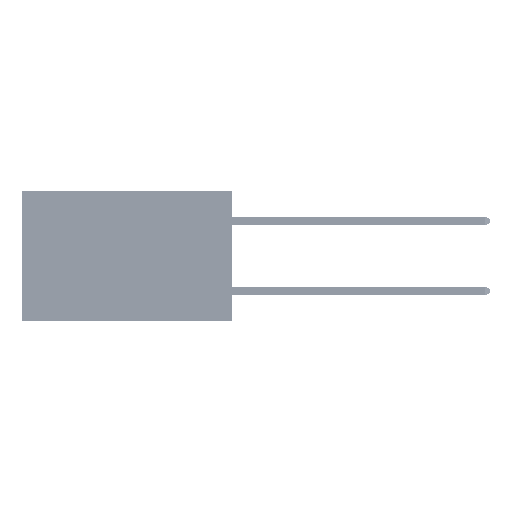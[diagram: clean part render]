
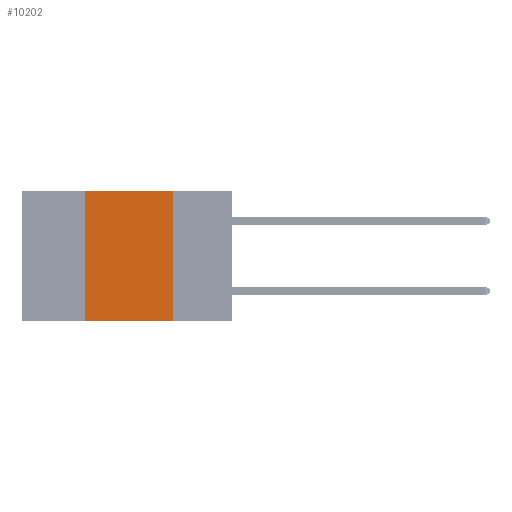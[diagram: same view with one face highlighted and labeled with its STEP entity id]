
A CAD part, left-side view. The second image highlights one B-rep face of the part: STEP entity #10202.
In plain terms, the highlighted planar face has unit normal (-1, 0, 0).
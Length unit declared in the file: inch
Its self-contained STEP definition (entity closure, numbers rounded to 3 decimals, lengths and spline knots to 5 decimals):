
#635 = VECTOR ( 'NONE', #24639, 39.37008 ) ;
#2583 = EDGE_CURVE ( 'NONE', #3185, #27269, #31973, .T. ) ;
#2627 = ORIENTED_EDGE ( 'NONE', *, *, #12925, .F. ) ;
#2880 = DIRECTION ( 'NONE',  ( 1., 0., 0. ) ) ;
#3185 = VERTEX_POINT ( 'NONE', #38075 ) ;
#7479 = VECTOR ( 'NONE', #16500, 39.37008 ) ;
#10202 = ADVANCED_FACE ( 'NONE', ( #27167 ), #19572, .F. ) ;
#11979 = DIRECTION ( 'NONE',  ( 0., 0., 1. ) ) ;
#12925 = EDGE_CURVE ( 'NONE', #47387, #3185, #31853, .T. ) ;
#13907 = EDGE_CURVE ( 'NONE', #27269, #35671, #40503, .T. ) ;
#14994 = ORIENTED_EDGE ( 'NONE', *, *, #13907, .F. ) ;
#16241 = LINE ( 'NONE', #47823, #22412 ) ;
#16500 = DIRECTION ( 'NONE',  ( 0., 0., -1. ) ) ;
#18069 = VECTOR ( 'NONE', #11979, 39.37008 ) ;
#19572 = PLANE ( 'NONE',  #29529 ) ;
#22138 = EDGE_CURVE ( 'NONE', #47387, #35671, #16241, .T. ) ;
#22412 = VECTOR ( 'NONE', #44181, 39.37008 ) ;
#24071 = CARTESIAN_POINT ( 'NONE',  ( 0., 0.17, -0.37 ) ) ;
#24639 = DIRECTION ( 'NONE',  ( 0., -1., 0. ) ) ;
#25840 = CARTESIAN_POINT ( 'NONE',  ( 0., 0.42, -0.37 ) ) ;
#27167 = FACE_OUTER_BOUND ( 'NONE', #39437, .T. ) ;
#27269 = VERTEX_POINT ( 'NONE', #37053 ) ;
#29529 = AXIS2_PLACEMENT_3D ( 'NONE', #51152, #2880, #46973 ) ;
#31725 = CARTESIAN_POINT ( 'NONE',  ( 0., 0.6, 0. ) ) ;
#31853 = LINE ( 'NONE', #47753, #18069 ) ;
#31973 = LINE ( 'NONE', #31725, #635 ) ;
#35671 = VERTEX_POINT ( 'NONE', #24071 ) ;
#37053 = CARTESIAN_POINT ( 'NONE',  ( 0., 0.17, 0. ) ) ;
#38075 = CARTESIAN_POINT ( 'NONE',  ( 0., 0.42, 0. ) ) ;
#39437 = EDGE_LOOP ( 'NONE', ( #14994, #48945, #2627, #48056 ) ) ;
#40503 = LINE ( 'NONE', #44424, #7479 ) ;
#44181 = DIRECTION ( 'NONE',  ( 0., -1., 0. ) ) ;
#44424 = CARTESIAN_POINT ( 'NONE',  ( 0., 0.17, 0. ) ) ;
#46973 = DIRECTION ( 'NONE',  ( 0., 0., -1. ) ) ;
#47387 = VERTEX_POINT ( 'NONE', #25840 ) ;
#47753 = CARTESIAN_POINT ( 'NONE',  ( 0., 0.42, 0. ) ) ;
#47823 = CARTESIAN_POINT ( 'NONE',  ( 0., 0.6, -0.37 ) ) ;
#48056 = ORIENTED_EDGE ( 'NONE', *, *, #22138, .T. ) ;
#48945 = ORIENTED_EDGE ( 'NONE', *, *, #2583, .F. ) ;
#51152 = CARTESIAN_POINT ( 'NONE',  ( 0., 0.6, 0. ) ) ;
